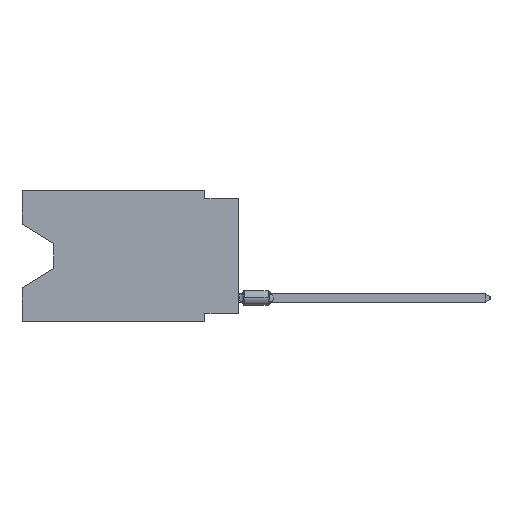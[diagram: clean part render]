
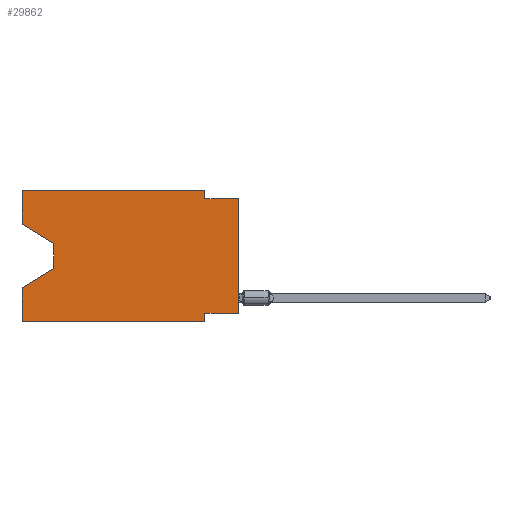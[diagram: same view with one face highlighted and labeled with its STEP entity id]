
A CAD part, left-side view. The second image highlights one B-rep face of the part: STEP entity #29862.
In plain terms, the highlighted planar face has unit normal (-1, 0, 0).
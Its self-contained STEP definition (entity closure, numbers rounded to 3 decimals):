
#21 = ORIENTED_EDGE ( 'NONE', *, *, #22705, .T. ) ;
#85 = EDGE_LOOP ( 'NONE', ( #7843, #3081, #21, #18389, #18090, #20217, #6273, #20562, #11294, #27416, #25199, #8793 ) ) ;
#164 = VECTOR ( 'NONE', #10652, 1000. ) ;
#278 = VERTEX_POINT ( 'NONE', #21456 ) ;
#301 = DIRECTION ( 'NONE',  ( 1., 0., 0. ) ) ;
#320 = CARTESIAN_POINT ( 'NONE',  ( 0., 0., 0. ) ) ;
#481 = LINE ( 'NONE', #25253, #12196 ) ;
#1137 = EDGE_CURVE ( 'NONE', #21147, #1339, #6064, .T. ) ;
#1216 = VERTEX_POINT ( 'NONE', #20106 ) ;
#1339 = VERTEX_POINT ( 'NONE', #7480 ) ;
#2173 = EDGE_CURVE ( 'NONE', #5347, #6292, #17719, .T. ) ;
#2612 = EDGE_CURVE ( 'NONE', #19443, #5347, #7324, .T. ) ;
#3081 = ORIENTED_EDGE ( 'NONE', *, *, #22501, .T. ) ;
#3435 = CARTESIAN_POINT ( 'NONE',  ( 0., 16.383, 0. ) ) ;
#4197 = VECTOR ( 'NONE', #10290, 1000. ) ;
#4282 = VERTEX_POINT ( 'NONE', #25727 ) ;
#5347 = VERTEX_POINT ( 'NONE', #24033 ) ;
#5428 = CARTESIAN_POINT ( 'NONE',  ( 0., 16.383, -9.906 ) ) ;
#5447 = DIRECTION ( 'NONE',  ( 0., 0., -1. ) ) ;
#6064 = LINE ( 'NONE', #3435, #164 ) ;
#6273 = ORIENTED_EDGE ( 'NONE', *, *, #2612, .F. ) ;
#6292 = VERTEX_POINT ( 'NONE', #18407 ) ;
#6780 = CARTESIAN_POINT ( 'NONE',  ( 0., 13.97, -4.013 ) ) ;
#7145 = EDGE_CURVE ( 'NONE', #19443, #278, #15171, .T. ) ;
#7323 = LINE ( 'NONE', #6780, #15580 ) ;
#7324 = LINE ( 'NONE', #18026, #12065 ) ;
#7480 = CARTESIAN_POINT ( 'NONE',  ( 0., 2.54, 0. ) ) ;
#7843 = ORIENTED_EDGE ( 'NONE', *, *, #21295, .T. ) ;
#8095 = LINE ( 'NONE', #29493, #11148 ) ;
#8793 = ORIENTED_EDGE ( 'NONE', *, *, #16081, .F. ) ;
#8975 = LINE ( 'NONE', #20017, #23521 ) ;
#10290 = DIRECTION ( 'NONE',  ( 0., 0., 1. ) ) ;
#10521 = VECTOR ( 'NONE', #11628, 1000. ) ;
#10652 = DIRECTION ( 'NONE',  ( 0., -1., 0. ) ) ;
#11148 = VECTOR ( 'NONE', #5447, 1000. ) ;
#11209 = DIRECTION ( 'NONE',  ( 0., 0.855, -0.519 ) ) ;
#11294 = ORIENTED_EDGE ( 'NONE', *, *, #17194, .F. ) ;
#11628 = DIRECTION ( 'NONE',  ( 0., -1., 0. ) ) ;
#11693 = LINE ( 'NONE', #12578, #29187 ) ;
#11748 = VECTOR ( 'NONE', #24479, 1000. ) ;
#12065 = VECTOR ( 'NONE', #13092, 1000. ) ;
#12196 = VECTOR ( 'NONE', #11209, 1000. ) ;
#12578 = CARTESIAN_POINT ( 'NONE',  ( 0., 16.383, -2.546 ) ) ;
#12970 = CARTESIAN_POINT ( 'NONE',  ( 0., 16.383, -2.546 ) ) ;
#13092 = DIRECTION ( 'NONE',  ( 0., 1., 0. ) ) ;
#13658 = FACE_OUTER_BOUND ( 'NONE', #85, .T. ) ;
#15123 = DIRECTION ( 'NONE',  ( 0., 0., 1. ) ) ;
#15171 = LINE ( 'NONE', #320, #20478 ) ;
#15403 = CARTESIAN_POINT ( 'NONE',  ( 0., 16.383, 0. ) ) ;
#15580 = VECTOR ( 'NONE', #18023, 1000. ) ;
#16081 = EDGE_CURVE ( 'NONE', #25870, #21147, #34181, .T. ) ;
#17109 = LINE ( 'NONE', #30278, #11748 ) ;
#17194 = EDGE_CURVE ( 'NONE', #23560, #278, #20406, .T. ) ;
#17719 = LINE ( 'NONE', #28420, #28283 ) ;
#18023 = DIRECTION ( 'NONE',  ( 0., 0., -1. ) ) ;
#18026 = CARTESIAN_POINT ( 'NONE',  ( 0., 0., -9.271 ) ) ;
#18090 = ORIENTED_EDGE ( 'NONE', *, *, #28426, .T. ) ;
#18335 = CARTESIAN_POINT ( 'NONE',  ( 0., 16.383, -7.36 ) ) ;
#18389 = ORIENTED_EDGE ( 'NONE', *, *, #18747, .F. ) ;
#18407 = CARTESIAN_POINT ( 'NONE',  ( 0., 2.54, -9.906 ) ) ;
#18747 = EDGE_CURVE ( 'NONE', #21847, #34502, #8975, .T. ) ;
#19443 = VERTEX_POINT ( 'NONE', #31467 ) ;
#19567 = EDGE_CURVE ( 'NONE', #1339, #23560, #8095, .T. ) ;
#20017 = CARTESIAN_POINT ( 'NONE',  ( 0., 16.383, 0. ) ) ;
#20106 = CARTESIAN_POINT ( 'NONE',  ( 0., 13.97, -5.893 ) ) ;
#20217 = ORIENTED_EDGE ( 'NONE', *, *, #2173, .F. ) ;
#20406 = LINE ( 'NONE', #22856, #10521 ) ;
#20478 = VECTOR ( 'NONE', #23236, 1000. ) ;
#20562 = ORIENTED_EDGE ( 'NONE', *, *, #7145, .T. ) ;
#20694 = CARTESIAN_POINT ( 'NONE',  ( 0., 2.54, -0.635 ) ) ;
#20697 = DIRECTION ( 'NONE',  ( 0., 0., -1. ) ) ;
#21147 = VERTEX_POINT ( 'NONE', #23668 ) ;
#21295 = EDGE_CURVE ( 'NONE', #25870, #4282, #11693, .T. ) ;
#21456 = CARTESIAN_POINT ( 'NONE',  ( 0., 0., -0.635 ) ) ;
#21847 = VERTEX_POINT ( 'NONE', #5428 ) ;
#22501 = EDGE_CURVE ( 'NONE', #4282, #1216, #7323, .T. ) ;
#22705 = EDGE_CURVE ( 'NONE', #1216, #34502, #481, .T. ) ;
#22856 = CARTESIAN_POINT ( 'NONE',  ( 0., 0., -0.635 ) ) ;
#23236 = DIRECTION ( 'NONE',  ( 0., 0., 1. ) ) ;
#23521 = VECTOR ( 'NONE', #15123, 1000. ) ;
#23560 = VERTEX_POINT ( 'NONE', #20694 ) ;
#23668 = CARTESIAN_POINT ( 'NONE',  ( 0., 16.383, 0. ) ) ;
#24033 = CARTESIAN_POINT ( 'NONE',  ( 0., 2.54, -9.271 ) ) ;
#24361 = CARTESIAN_POINT ( 'NONE',  ( 0., 16.383, 0. ) ) ;
#24479 = DIRECTION ( 'NONE',  ( 0., -1., 0. ) ) ;
#25061 = DIRECTION ( 'NONE',  ( 0., 0., -1. ) ) ;
#25199 = ORIENTED_EDGE ( 'NONE', *, *, #1137, .F. ) ;
#25253 = CARTESIAN_POINT ( 'NONE',  ( 0., 13.97, -5.893 ) ) ;
#25727 = CARTESIAN_POINT ( 'NONE',  ( 0., 13.97, -4.013 ) ) ;
#25870 = VERTEX_POINT ( 'NONE', #12970 ) ;
#27416 = ORIENTED_EDGE ( 'NONE', *, *, #19567, .F. ) ;
#28283 = VECTOR ( 'NONE', #20697, 1000. ) ;
#28420 = CARTESIAN_POINT ( 'NONE',  ( 0., 2.54, -9.906 ) ) ;
#28426 = EDGE_CURVE ( 'NONE', #21847, #6292, #17109, .T. ) ;
#29187 = VECTOR ( 'NONE', #30656, 1000. ) ;
#29493 = CARTESIAN_POINT ( 'NONE',  ( 0., 2.54, 0. ) ) ;
#29862 = ADVANCED_FACE ( 'NONE', ( #13658 ), #32270, .F. ) ;
#30278 = CARTESIAN_POINT ( 'NONE',  ( 0., 16.383, -9.906 ) ) ;
#30656 = DIRECTION ( 'NONE',  ( 0., -0.855, -0.519 ) ) ;
#31467 = CARTESIAN_POINT ( 'NONE',  ( 0., 0., -9.271 ) ) ;
#32270 = PLANE ( 'NONE',  #34249 ) ;
#34181 = LINE ( 'NONE', #15403, #4197 ) ;
#34249 = AXIS2_PLACEMENT_3D ( 'NONE', #24361, #301, #25061 ) ;
#34502 = VERTEX_POINT ( 'NONE', #18335 ) ;
